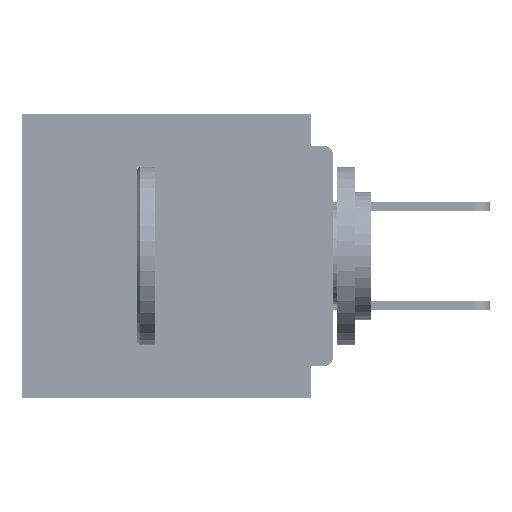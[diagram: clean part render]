
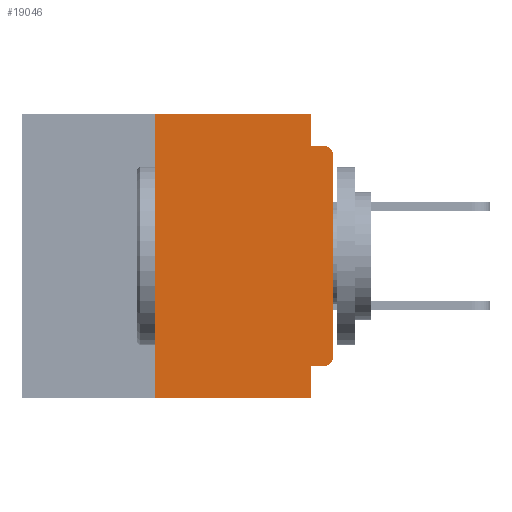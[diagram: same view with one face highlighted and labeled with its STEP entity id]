
A CAD part, left-side view. The second image highlights one B-rep face of the part: STEP entity #19046.
In plain terms, the highlighted planar face has unit normal (-1, 0, 0).
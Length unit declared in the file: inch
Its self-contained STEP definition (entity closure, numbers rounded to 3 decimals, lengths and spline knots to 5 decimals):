
#1252 = CARTESIAN_POINT ( 'NONE',  ( 0., 0.015, -0.045 ) ) ;
#1702 = ORIENTED_EDGE ( 'NONE', *, *, #19533, .F. ) ;
#3143 = DIRECTION ( 'NONE',  ( 0., 1., 0. ) ) ;
#3261 = CARTESIAN_POINT ( 'NONE',  ( 0., 0., -0.34 ) ) ;
#3426 = CIRCLE ( 'NONE', #55281, 0.015 ) ;
#3783 = CARTESIAN_POINT ( 'NONE',  ( 0., 0.031, -0.4 ) ) ;
#4930 = LINE ( 'NONE', #6493, #28728 ) ;
#5263 = LINE ( 'NONE', #44080, #16428 ) ;
#6493 = CARTESIAN_POINT ( 'NONE',  ( 0., 0.437, -0.4 ) ) ;
#7373 = CARTESIAN_POINT ( 'NONE',  ( 0., 0.031, -0.4 ) ) ;
#7896 = EDGE_CURVE ( 'NONE', #15371, #19845, #46680, .T. ) ;
#8352 = DIRECTION ( 'NONE',  ( 0., 0., -1. ) ) ;
#10945 = DIRECTION ( 'NONE',  ( 0., 0., -1. ) ) ;
#11081 = VERTEX_POINT ( 'NONE', #50942 ) ;
#11398 = LINE ( 'NONE', #52602, #24061 ) ;
#12025 = VECTOR ( 'NONE', #33777, 39.37008 ) ;
#13549 = LINE ( 'NONE', #33976, #12025 ) ;
#13806 = EDGE_CURVE ( 'NONE', #61244, #20974, #5263, .T. ) ;
#14096 = CARTESIAN_POINT ( 'NONE',  ( 0., 0.015, -0.355 ) ) ;
#14549 = CARTESIAN_POINT ( 'NONE',  ( 0., 0.25, 0. ) ) ;
#15371 = VERTEX_POINT ( 'NONE', #23065 ) ;
#15760 = CARTESIAN_POINT ( 'NONE',  ( 0., 0.031, 0. ) ) ;
#16428 = VECTOR ( 'NONE', #48845, 39.37008 ) ;
#17186 = VERTEX_POINT ( 'NONE', #23751 ) ;
#17636 = EDGE_CURVE ( 'NONE', #59699, #25837, #51096, .T. ) ;
#17871 = DIRECTION ( 'NONE',  ( -1., 0., 0. ) ) ;
#19046 = ADVANCED_FACE ( 'NONE', ( #33170 ), #22913, .F. ) ;
#19533 = EDGE_CURVE ( 'NONE', #25837, #27053, #42749, .T. ) ;
#19845 = VERTEX_POINT ( 'NONE', #1252 ) ;
#20974 = VERTEX_POINT ( 'NONE', #50486 ) ;
#22432 = ORIENTED_EDGE ( 'NONE', *, *, #51282, .F. ) ;
#22913 = PLANE ( 'NONE',  #24412 ) ;
#23065 = CARTESIAN_POINT ( 'NONE',  ( 0., 0., -0.06 ) ) ;
#23751 = CARTESIAN_POINT ( 'NONE',  ( 0., 0.031, -0.045 ) ) ;
#23855 = EDGE_CURVE ( 'NONE', #59699, #36532, #3426, .T. ) ;
#24061 = VECTOR ( 'NONE', #38275, 39.37008 ) ;
#24412 = AXIS2_PLACEMENT_3D ( 'NONE', #56157, #60954, #32474 ) ;
#24541 = ORIENTED_EDGE ( 'NONE', *, *, #31541, .F. ) ;
#24554 = DIRECTION ( 'NONE',  ( 0., 0., 1. ) ) ;
#24776 = ORIENTED_EDGE ( 'NONE', *, *, #13806, .F. ) ;
#25812 = VECTOR ( 'NONE', #3143, 39.37008 ) ;
#25837 = VERTEX_POINT ( 'NONE', #38424 ) ;
#25891 = ORIENTED_EDGE ( 'NONE', *, *, #17636, .F. ) ;
#27053 = VERTEX_POINT ( 'NONE', #7373 ) ;
#28074 = DIRECTION ( 'NONE',  ( -1., 0., 0. ) ) ;
#28145 = LINE ( 'NONE', #15760, #51914 ) ;
#28728 = VECTOR ( 'NONE', #39721, 39.37008 ) ;
#30997 = EDGE_CURVE ( 'NONE', #17186, #19845, #13549, .T. ) ;
#31302 = LINE ( 'NONE', #48222, #55073 ) ;
#31541 = EDGE_CURVE ( 'NONE', #11081, #61244, #31302, .T. ) ;
#31609 = CARTESIAN_POINT ( 'NONE',  ( 0., 0., -0.355 ) ) ;
#32474 = DIRECTION ( 'NONE',  ( 0., 0., -1. ) ) ;
#33170 = FACE_OUTER_BOUND ( 'NONE', #59470, .T. ) ;
#33777 = DIRECTION ( 'NONE',  ( 0., -1., 0. ) ) ;
#33976 = CARTESIAN_POINT ( 'NONE',  ( 0., 0., -0.045 ) ) ;
#36532 = VERTEX_POINT ( 'NONE', #3261 ) ;
#37139 = ORIENTED_EDGE ( 'NONE', *, *, #30997, .F. ) ;
#38275 = DIRECTION ( 'NONE',  ( 0., 0., 1. ) ) ;
#38424 = CARTESIAN_POINT ( 'NONE',  ( 0., 0.031, -0.355 ) ) ;
#39721 = DIRECTION ( 'NONE',  ( 0., -1., 0. ) ) ;
#42749 = LINE ( 'NONE', #3783, #52423 ) ;
#44080 = CARTESIAN_POINT ( 'NONE',  ( 0., 0.437, 0. ) ) ;
#46177 = ORIENTED_EDGE ( 'NONE', *, *, #53600, .T. ) ;
#46309 = CARTESIAN_POINT ( 'NONE',  ( 0., 0.015, -0.06 ) ) ;
#46680 = CIRCLE ( 'NONE', #50410, 0.015 ) ;
#48222 = CARTESIAN_POINT ( 'NONE',  ( 0., 0.25, -0.4 ) ) ;
#48845 = DIRECTION ( 'NONE',  ( 0., -1., 0. ) ) ;
#50410 = AXIS2_PLACEMENT_3D ( 'NONE', #46309, #17871, #51094 ) ;
#50486 = CARTESIAN_POINT ( 'NONE',  ( 0., 0.031, 0. ) ) ;
#50942 = CARTESIAN_POINT ( 'NONE',  ( 0., 0.25, -0.4 ) ) ;
#51094 = DIRECTION ( 'NONE',  ( 0., 0., -1. ) ) ;
#51096 = LINE ( 'NONE', #31609, #25812 ) ;
#51282 = EDGE_CURVE ( 'NONE', #20974, #17186, #28145, .T. ) ;
#51914 = VECTOR ( 'NONE', #10945, 39.37008 ) ;
#52423 = VECTOR ( 'NONE', #8352, 39.37008 ) ;
#52602 = CARTESIAN_POINT ( 'NONE',  ( 0., 0., 0. ) ) ;
#53409 = ORIENTED_EDGE ( 'NONE', *, *, #23855, .T. ) ;
#53600 = EDGE_CURVE ( 'NONE', #36532, #15371, #11398, .T. ) ;
#55073 = VECTOR ( 'NONE', #24554, 39.37008 ) ;
#55281 = AXIS2_PLACEMENT_3D ( 'NONE', #56516, #28074, #61330 ) ;
#56157 = CARTESIAN_POINT ( 'NONE',  ( 0., 0.437, 0. ) ) ;
#56516 = CARTESIAN_POINT ( 'NONE',  ( 0., 0.015, -0.34 ) ) ;
#57236 = ORIENTED_EDGE ( 'NONE', *, *, #7896, .T. ) ;
#57554 = EDGE_CURVE ( 'NONE', #11081, #27053, #4930, .T. ) ;
#58928 = ORIENTED_EDGE ( 'NONE', *, *, #57554, .T. ) ;
#59470 = EDGE_LOOP ( 'NONE', ( #46177, #57236, #37139, #22432, #24776, #24541, #58928, #1702, #25891, #53409 ) ) ;
#59699 = VERTEX_POINT ( 'NONE', #14096 ) ;
#60954 = DIRECTION ( 'NONE',  ( 1., 0., 0. ) ) ;
#61244 = VERTEX_POINT ( 'NONE', #14549 ) ;
#61330 = DIRECTION ( 'NONE',  ( 0., 0., -1. ) ) ;
